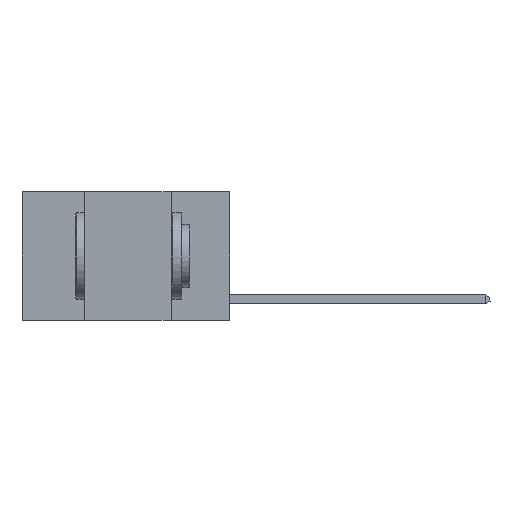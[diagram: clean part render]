
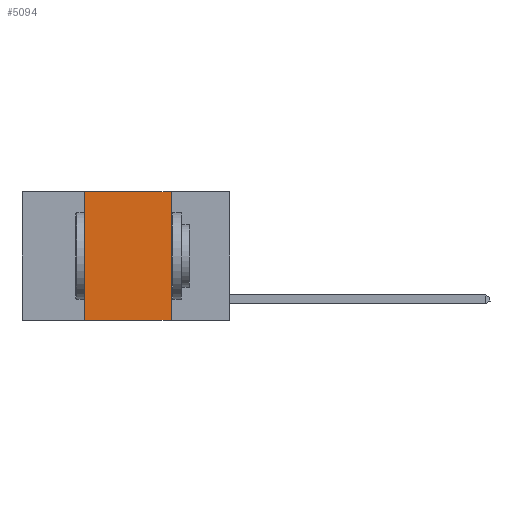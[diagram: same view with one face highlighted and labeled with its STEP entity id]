
A CAD part, left-side view. The second image highlights one B-rep face of the part: STEP entity #5094.
In plain terms, the highlighted planar face has unit normal (-1, 0, 0).
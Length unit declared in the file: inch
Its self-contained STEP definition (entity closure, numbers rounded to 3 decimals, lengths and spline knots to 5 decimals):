
#157 = CARTESIAN_POINT ( 'NONE',  ( 0., 0.17, 0. ) ) ;
#984 = ORIENTED_EDGE ( 'NONE', *, *, #11980, .F. ) ;
#1691 = VERTEX_POINT ( 'NONE', #17041 ) ;
#2812 = CARTESIAN_POINT ( 'NONE',  ( 0., 0.42, 0. ) ) ;
#3161 = DIRECTION ( 'NONE',  ( 0., 0., -1. ) ) ;
#3305 = DIRECTION ( 'NONE',  ( 1., 0., 0. ) ) ;
#3556 = PLANE ( 'NONE',  #10028 ) ;
#3768 = CARTESIAN_POINT ( 'NONE',  ( 0., 0.6, 0. ) ) ;
#3923 = EDGE_CURVE ( 'NONE', #1691, #13913, #10160, .T. ) ;
#4284 = VERTEX_POINT ( 'NONE', #2812 ) ;
#4748 = ORIENTED_EDGE ( 'NONE', *, *, #3923, .T. ) ;
#5094 = ADVANCED_FACE ( 'NONE', ( #8879 ), #3556, .F. ) ;
#5614 = EDGE_LOOP ( 'NONE', ( #14542, #7588, #984, #4748 ) ) ;
#5664 = CARTESIAN_POINT ( 'NONE',  ( 0., 0.42, 0. ) ) ;
#6001 = CARTESIAN_POINT ( 'NONE',  ( 0., 0.17, 0. ) ) ;
#7003 = LINE ( 'NONE', #5664, #10216 ) ;
#7395 = CARTESIAN_POINT ( 'NONE',  ( 0., 0.6, 0. ) ) ;
#7396 = DIRECTION ( 'NONE',  ( 0., 0., -1. ) ) ;
#7588 = ORIENTED_EDGE ( 'NONE', *, *, #17372, .F. ) ;
#8035 = VERTEX_POINT ( 'NONE', #157 ) ;
#8787 = DIRECTION ( 'NONE',  ( 0., -1., 0. ) ) ;
#8879 = FACE_OUTER_BOUND ( 'NONE', #5614, .T. ) ;
#9402 = LINE ( 'NONE', #7395, #16366 ) ;
#10028 = AXIS2_PLACEMENT_3D ( 'NONE', #3768, #3305, #3161 ) ;
#10160 = LINE ( 'NONE', #12362, #17192 ) ;
#10216 = VECTOR ( 'NONE', #18110, 39.37008 ) ;
#10608 = VECTOR ( 'NONE', #7396, 39.37008 ) ;
#11033 = LINE ( 'NONE', #6001, #10608 ) ;
#11980 = EDGE_CURVE ( 'NONE', #1691, #4284, #7003, .T. ) ;
#12362 = CARTESIAN_POINT ( 'NONE',  ( 0., 0.6, -0.37 ) ) ;
#12790 = EDGE_CURVE ( 'NONE', #8035, #13913, #11033, .T. ) ;
#12830 = CARTESIAN_POINT ( 'NONE',  ( 0., 0.17, -0.37 ) ) ;
#13913 = VERTEX_POINT ( 'NONE', #12830 ) ;
#14542 = ORIENTED_EDGE ( 'NONE', *, *, #12790, .F. ) ;
#15911 = DIRECTION ( 'NONE',  ( 0., -1., 0. ) ) ;
#16366 = VECTOR ( 'NONE', #8787, 39.37008 ) ;
#17041 = CARTESIAN_POINT ( 'NONE',  ( 0., 0.42, -0.37 ) ) ;
#17192 = VECTOR ( 'NONE', #15911, 39.37008 ) ;
#17372 = EDGE_CURVE ( 'NONE', #4284, #8035, #9402, .T. ) ;
#18110 = DIRECTION ( 'NONE',  ( 0., 0., 1. ) ) ;
